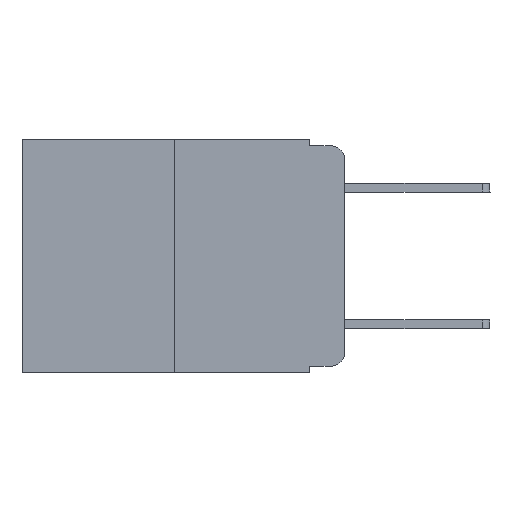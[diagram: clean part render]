
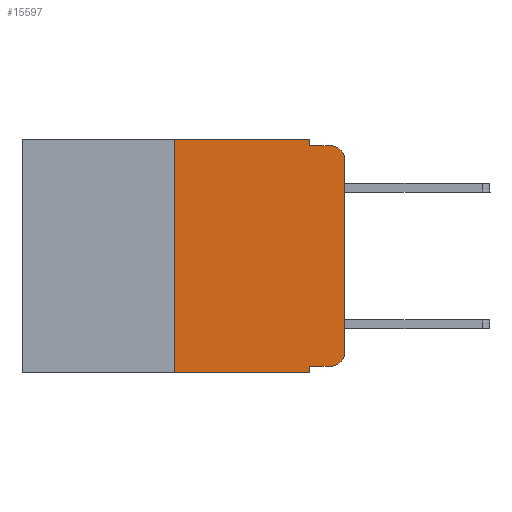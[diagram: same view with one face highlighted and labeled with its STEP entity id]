
A CAD part, left-side view. The second image highlights one B-rep face of the part: STEP entity #15597.
In plain terms, the highlighted planar face has unit normal (-1, 0, 0).
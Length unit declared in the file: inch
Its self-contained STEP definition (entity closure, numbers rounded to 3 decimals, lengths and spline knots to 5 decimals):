
#57 = CARTESIAN_POINT ( 'NONE',  ( 0., 0.473, -0.343 ) ) ;
#217 = VERTEX_POINT ( 'NONE', #19329 ) ;
#307 = AXIS2_PLACEMENT_3D ( 'NONE', #14471, #1222, #10132 ) ;
#407 = DIRECTION ( 'NONE',  ( 0., 0., -1. ) ) ;
#940 = EDGE_CURVE ( 'NONE', #217, #1410, #3690, .T. ) ;
#1076 = VERTEX_POINT ( 'NONE', #1431 ) ;
#1222 = DIRECTION ( 'NONE',  ( 1., 0., 0. ) ) ;
#1344 = ORIENTED_EDGE ( 'NONE', *, *, #15345, .T. ) ;
#1404 = CARTESIAN_POINT ( 'NONE',  ( 0., 0.02, -0.333 ) ) ;
#1410 = VERTEX_POINT ( 'NONE', #16490 ) ;
#1431 = CARTESIAN_POINT ( 'NONE',  ( 0., 0.051, 0. ) ) ;
#1537 = EDGE_CURVE ( 'NONE', #10194, #17887, #6179, .T. ) ;
#1729 = ORIENTED_EDGE ( 'NONE', *, *, #13508, .T. ) ;
#1779 = VECTOR ( 'NONE', #18701, 39.37008 ) ;
#1949 = LINE ( 'NONE', #10952, #6628 ) ;
#1986 = EDGE_CURVE ( 'NONE', #11845, #217, #4459, .T. ) ;
#2224 = CARTESIAN_POINT ( 'NONE',  ( 0., 0.051, -0.333 ) ) ;
#2289 = DIRECTION ( 'NONE',  ( 0., -1., 0. ) ) ;
#2361 = CIRCLE ( 'NONE', #17381, 0.02 ) ;
#2774 = CARTESIAN_POINT ( 'NONE',  ( 0., 0.051, -0.01 ) ) ;
#2920 = LINE ( 'NONE', #5946, #19300 ) ;
#3284 = VECTOR ( 'NONE', #8857, 39.37008 ) ;
#3303 = ORIENTED_EDGE ( 'NONE', *, *, #16304, .F. ) ;
#3431 = VECTOR ( 'NONE', #7517, 39.37008 ) ;
#3690 = LINE ( 'NONE', #15664, #1779 ) ;
#4459 = CIRCLE ( 'NONE', #17947, 0.02 ) ;
#4609 = ORIENTED_EDGE ( 'NONE', *, *, #13460, .F. ) ;
#4794 = CARTESIAN_POINT ( 'NONE',  ( 0., 0.02, -0.313 ) ) ;
#5324 = EDGE_CURVE ( 'NONE', #5428, #1076, #13770, .T. ) ;
#5428 = VERTEX_POINT ( 'NONE', #11304 ) ;
#5717 = ORIENTED_EDGE ( 'NONE', *, *, #10741, .T. ) ;
#5889 = CARTESIAN_POINT ( 'NONE',  ( 0., 0.051, -0.01 ) ) ;
#5905 = ORIENTED_EDGE ( 'NONE', *, *, #1986, .T. ) ;
#5946 = CARTESIAN_POINT ( 'NONE',  ( 0., 0.051, -0.333 ) ) ;
#6179 = LINE ( 'NONE', #5889, #3284 ) ;
#6628 = VECTOR ( 'NONE', #9379, 39.37008 ) ;
#7517 = DIRECTION ( 'NONE',  ( 0., -1., 0. ) ) ;
#7703 = ORIENTED_EDGE ( 'NONE', *, *, #1537, .F. ) ;
#8628 = DIRECTION ( 'NONE',  ( 0., -1., 0. ) ) ;
#8857 = DIRECTION ( 'NONE',  ( 0., -1., 0. ) ) ;
#9379 = DIRECTION ( 'NONE',  ( 0., 0., -1. ) ) ;
#9596 = CARTESIAN_POINT ( 'NONE',  ( 0., 0.25, 0. ) ) ;
#10077 = CARTESIAN_POINT ( 'NONE',  ( 0., 0.051, 0. ) ) ;
#10132 = DIRECTION ( 'NONE',  ( 0., 0., -1. ) ) ;
#10194 = VERTEX_POINT ( 'NONE', #2774 ) ;
#10384 = DIRECTION ( 'NONE',  ( -1., 0., 0. ) ) ;
#10385 = VERTEX_POINT ( 'NONE', #11206 ) ;
#10741 = EDGE_CURVE ( 'NONE', #1410, #17887, #2361, .T. ) ;
#10839 = LINE ( 'NONE', #57, #3431 ) ;
#10937 = EDGE_LOOP ( 'NONE', ( #11368, #5717, #7703, #17522, #16903, #3303, #1344, #4609, #1729, #5905 ) ) ;
#10952 = CARTESIAN_POINT ( 'NONE',  ( 0., 0.051, 0. ) ) ;
#11206 = CARTESIAN_POINT ( 'NONE',  ( 0., 0.25, -0.343 ) ) ;
#11241 = VERTEX_POINT ( 'NONE', #17137 ) ;
#11304 = CARTESIAN_POINT ( 'NONE',  ( 0., 0.25, 0. ) ) ;
#11368 = ORIENTED_EDGE ( 'NONE', *, *, #940, .T. ) ;
#11845 = VERTEX_POINT ( 'NONE', #1404 ) ;
#11868 = DIRECTION ( 'NONE',  ( 0., 0., -1. ) ) ;
#13199 = FACE_OUTER_BOUND ( 'NONE', #10937, .T. ) ;
#13460 = EDGE_CURVE ( 'NONE', #18170, #11241, #16064, .T. ) ;
#13508 = EDGE_CURVE ( 'NONE', #18170, #11845, #2920, .T. ) ;
#13770 = LINE ( 'NONE', #15433, #16632 ) ;
#13948 = DIRECTION ( 'NONE',  ( -1., 0., 0. ) ) ;
#14134 = VECTOR ( 'NONE', #17407, 39.37008 ) ;
#14471 = CARTESIAN_POINT ( 'NONE',  ( 0., 0.473, 0. ) ) ;
#14486 = LINE ( 'NONE', #9596, #14134 ) ;
#14662 = PLANE ( 'NONE',  #307 ) ;
#15181 = CARTESIAN_POINT ( 'NONE',  ( 0., 0.02, -0.01 ) ) ;
#15345 = EDGE_CURVE ( 'NONE', #10385, #11241, #10839, .T. ) ;
#15433 = CARTESIAN_POINT ( 'NONE',  ( 0., 0.473, 0. ) ) ;
#15597 = ADVANCED_FACE ( 'NONE', ( #13199 ), #14662, .F. ) ;
#15664 = CARTESIAN_POINT ( 'NONE',  ( 0., 0., 0. ) ) ;
#15855 = VECTOR ( 'NONE', #17736, 39.37008 ) ;
#16064 = LINE ( 'NONE', #10077, #15855 ) ;
#16304 = EDGE_CURVE ( 'NONE', #10385, #5428, #14486, .T. ) ;
#16490 = CARTESIAN_POINT ( 'NONE',  ( 0., 0., -0.03 ) ) ;
#16632 = VECTOR ( 'NONE', #2289, 39.37008 ) ;
#16872 = CARTESIAN_POINT ( 'NONE',  ( 0., 0.02, -0.03 ) ) ;
#16903 = ORIENTED_EDGE ( 'NONE', *, *, #5324, .F. ) ;
#17137 = CARTESIAN_POINT ( 'NONE',  ( 0., 0.051, -0.343 ) ) ;
#17381 = AXIS2_PLACEMENT_3D ( 'NONE', #16872, #13948, #407 ) ;
#17407 = DIRECTION ( 'NONE',  ( 0., 0., 1. ) ) ;
#17522 = ORIENTED_EDGE ( 'NONE', *, *, #19211, .F. ) ;
#17736 = DIRECTION ( 'NONE',  ( 0., 0., -1. ) ) ;
#17887 = VERTEX_POINT ( 'NONE', #15181 ) ;
#17947 = AXIS2_PLACEMENT_3D ( 'NONE', #4794, #10384, #11868 ) ;
#18170 = VERTEX_POINT ( 'NONE', #2224 ) ;
#18701 = DIRECTION ( 'NONE',  ( 0., 0., 1. ) ) ;
#19211 = EDGE_CURVE ( 'NONE', #1076, #10194, #1949, .T. ) ;
#19300 = VECTOR ( 'NONE', #8628, 39.37008 ) ;
#19329 = CARTESIAN_POINT ( 'NONE',  ( 0., 0., -0.313 ) ) ;
